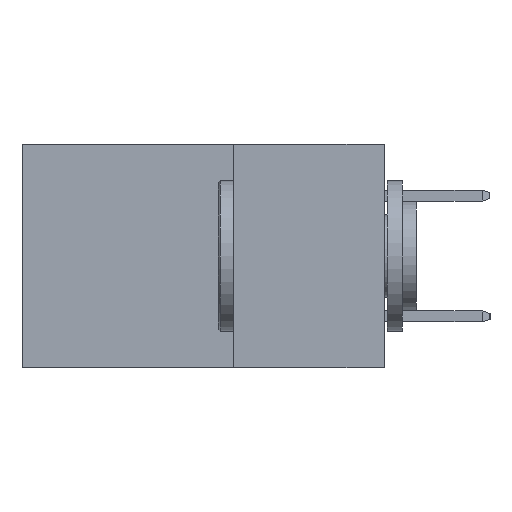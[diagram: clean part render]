
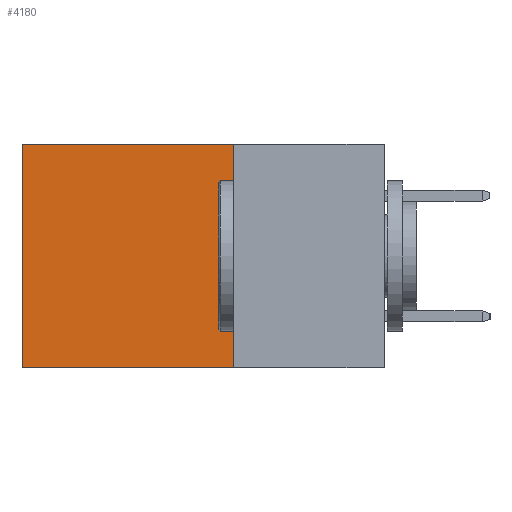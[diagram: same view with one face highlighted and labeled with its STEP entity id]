
A CAD part, left-side view. The second image highlights one B-rep face of the part: STEP entity #4180.
In plain terms, the highlighted planar face has unit normal (-1, 0, 0).
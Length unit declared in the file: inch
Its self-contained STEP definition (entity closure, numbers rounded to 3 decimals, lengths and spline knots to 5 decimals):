
#1292 = DIRECTION ( 'NONE',  ( 0., 1., 0. ) ) ;
#1410 = CARTESIAN_POINT ( 'NONE',  ( 0.2615, 0.25, 0. ) ) ;
#1447 = ORIENTED_EDGE ( 'NONE', *, *, #5499, .F. ) ;
#1858 = DIRECTION ( 'NONE',  ( 0., 0., -1. ) ) ;
#1927 = DIRECTION ( 'NONE',  ( 1., 0., 0. ) ) ;
#2086 = CARTESIAN_POINT ( 'NONE',  ( 0.2615, 0.25, -0.37 ) ) ;
#2124 = ORIENTED_EDGE ( 'NONE', *, *, #4209, .T. ) ;
#2179 = PLANE ( 'NONE',  #3058 ) ;
#2472 = CARTESIAN_POINT ( 'NONE',  ( 0.2615, 0.25, 0. ) ) ;
#3058 = AXIS2_PLACEMENT_3D ( 'NONE', #2086, #1927, #1858 ) ;
#3646 = EDGE_CURVE ( 'NONE', #7870, #9680, #6151, .T. ) ;
#4180 = ADVANCED_FACE ( 'NONE', ( #11518 ), #2179, .F. ) ;
#4209 = EDGE_CURVE ( 'NONE', #9193, #7870, #10832, .T. ) ;
#4559 = CARTESIAN_POINT ( 'NONE',  ( 0.2615, 0.6, 0. ) ) ;
#5402 = CARTESIAN_POINT ( 'NONE',  ( 0.2615, 0.25, -0.37 ) ) ;
#5486 = DIRECTION ( 'NONE',  ( 0., 1., 0. ) ) ;
#5499 = EDGE_CURVE ( 'NONE', #14875, #9680, #9397, .T. ) ;
#6021 = LINE ( 'NONE', #10589, #8780 ) ;
#6151 = LINE ( 'NONE', #13695, #8913 ) ;
#7174 = EDGE_CURVE ( 'NONE', #9193, #14875, #6021, .T. ) ;
#7588 = CARTESIAN_POINT ( 'NONE',  ( 0.2615, 0.25, -0.37 ) ) ;
#7870 = VERTEX_POINT ( 'NONE', #4559 ) ;
#8535 = ORIENTED_EDGE ( 'NONE', *, *, #3646, .T. ) ;
#8780 = VECTOR ( 'NONE', #10792, 39.37008 ) ;
#8913 = VECTOR ( 'NONE', #13459, 39.37008 ) ;
#9193 = VERTEX_POINT ( 'NONE', #2472 ) ;
#9397 = LINE ( 'NONE', #5402, #12365 ) ;
#9680 = VERTEX_POINT ( 'NONE', #12735 ) ;
#10475 = VECTOR ( 'NONE', #1292, 39.37008 ) ;
#10589 = CARTESIAN_POINT ( 'NONE',  ( 0.2615, 0.25, -0.37 ) ) ;
#10792 = DIRECTION ( 'NONE',  ( 0., 0., -1. ) ) ;
#10832 = LINE ( 'NONE', #1410, #10475 ) ;
#11488 = ORIENTED_EDGE ( 'NONE', *, *, #7174, .F. ) ;
#11518 = FACE_OUTER_BOUND ( 'NONE', #13356, .T. ) ;
#12365 = VECTOR ( 'NONE', #5486, 39.37008 ) ;
#12735 = CARTESIAN_POINT ( 'NONE',  ( 0.2615, 0.6, -0.37 ) ) ;
#13356 = EDGE_LOOP ( 'NONE', ( #8535, #1447, #11488, #2124 ) ) ;
#13459 = DIRECTION ( 'NONE',  ( 0., 0., -1. ) ) ;
#13695 = CARTESIAN_POINT ( 'NONE',  ( 0.2615, 0.6, -0.37 ) ) ;
#14875 = VERTEX_POINT ( 'NONE', #7588 ) ;
